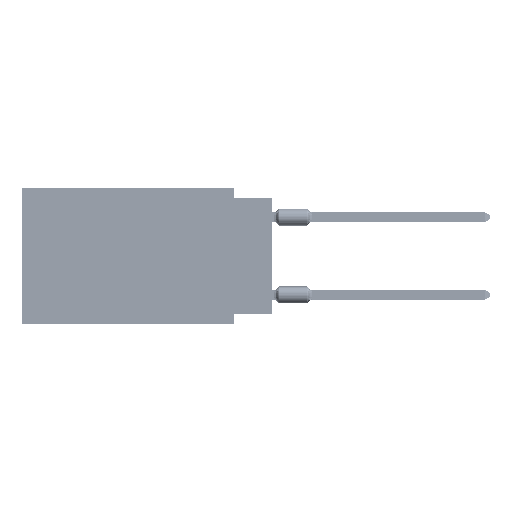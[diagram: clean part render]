
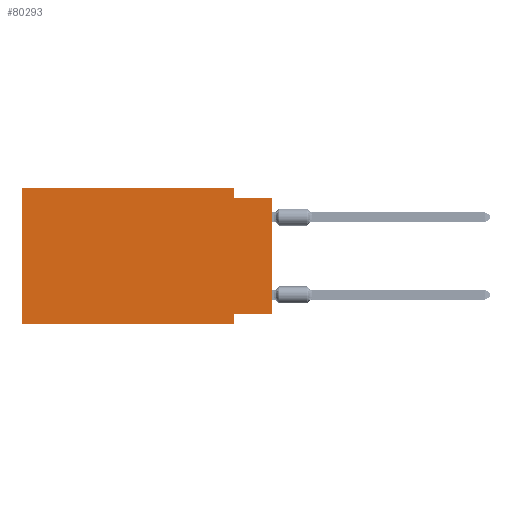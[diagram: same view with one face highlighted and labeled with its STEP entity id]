
A CAD part, left-side view. The second image highlights one B-rep face of the part: STEP entity #80293.
In plain terms, the highlighted planar face has unit normal (-1, 0, 0).
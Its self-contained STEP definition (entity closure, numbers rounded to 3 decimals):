
#221 = VECTOR ( 'NONE', #96902, 1000. ) ;
#2174 = VECTOR ( 'NONE', #97692, 1000. ) ;
#6761 = VERTEX_POINT ( 'NONE', #19589 ) ;
#8103 = VECTOR ( 'NONE', #70620, 1000. ) ;
#14086 = VERTEX_POINT ( 'NONE', #97853 ) ;
#14145 = EDGE_CURVE ( 'NONE', #23805, #6761, #61115, .T. ) ;
#17122 = CARTESIAN_POINT ( 'NONE',  ( 0., 16.383, -8.89 ) ) ;
#18074 = LINE ( 'NONE', #89787, #221 ) ;
#19589 = CARTESIAN_POINT ( 'NONE',  ( 0., 0., -0.635 ) ) ;
#19713 = LINE ( 'NONE', #30351, #54104 ) ;
#20325 = VERTEX_POINT ( 'NONE', #75668 ) ;
#23805 = VERTEX_POINT ( 'NONE', #88198 ) ;
#24097 = VECTOR ( 'NONE', #26695, 1000. ) ;
#25857 = ORIENTED_EDGE ( 'NONE', *, *, #102292, .F. ) ;
#26695 = DIRECTION ( 'NONE',  ( 0., -1., 0. ) ) ;
#28263 = DIRECTION ( 'NONE',  ( 0., 0., -1. ) ) ;
#29435 = LINE ( 'NONE', #92251, #42464 ) ;
#29451 = PLANE ( 'NONE',  #115308 ) ;
#30351 = CARTESIAN_POINT ( 'NONE',  ( 0., 0., -0.635 ) ) ;
#30402 = ORIENTED_EDGE ( 'NONE', *, *, #72761, .F. ) ;
#30609 = FACE_OUTER_BOUND ( 'NONE', #73069, .T. ) ;
#32565 = LINE ( 'NONE', #17122, #2174 ) ;
#32750 = ORIENTED_EDGE ( 'NONE', *, *, #60260, .T. ) ;
#37988 = DIRECTION ( 'NONE',  ( 0., 0., 1. ) ) ;
#38180 = VECTOR ( 'NONE', #37988, 1000. ) ;
#39143 = LINE ( 'NONE', #83614, #38180 ) ;
#40849 = EDGE_CURVE ( 'NONE', #14086, #113903, #72305, .T. ) ;
#42464 = VECTOR ( 'NONE', #28263, 1000. ) ;
#42532 = VECTOR ( 'NONE', #68549, 1000. ) ;
#46950 = DIRECTION ( 'NONE',  ( 0., -1., 0. ) ) ;
#48332 = CARTESIAN_POINT ( 'NONE',  ( 0., 16.383, -8.89 ) ) ;
#49326 = ORIENTED_EDGE ( 'NONE', *, *, #14145, .T. ) ;
#52803 = CARTESIAN_POINT ( 'NONE',  ( 0., 0., 0. ) ) ;
#54104 = VECTOR ( 'NONE', #46950, 1000. ) ;
#54745 = VERTEX_POINT ( 'NONE', #115375 ) ;
#60170 = DIRECTION ( 'NONE',  ( 0., 0., -1. ) ) ;
#60260 = EDGE_CURVE ( 'NONE', #61807, #54745, #32565, .T. ) ;
#60377 = VERTEX_POINT ( 'NONE', #100279 ) ;
#61115 = LINE ( 'NONE', #52803, #8103 ) ;
#61807 = VERTEX_POINT ( 'NONE', #48332 ) ;
#65578 = DIRECTION ( 'NONE',  ( 1., 0., 0. ) ) ;
#66745 = CARTESIAN_POINT ( 'NONE',  ( 0., 16.383, 0. ) ) ;
#68549 = DIRECTION ( 'NONE',  ( 0., 1., 0. ) ) ;
#70308 = LINE ( 'NONE', #106430, #42532 ) ;
#70620 = DIRECTION ( 'NONE',  ( 0., 0., 1. ) ) ;
#72305 = LINE ( 'NONE', #107853, #24097 ) ;
#72537 = ORIENTED_EDGE ( 'NONE', *, *, #96953, .F. ) ;
#72761 = EDGE_CURVE ( 'NONE', #23805, #60377, #70308, .T. ) ;
#73069 = EDGE_LOOP ( 'NONE', ( #49326, #25857, #72537, #75084, #108240, #32750, #100938, #30402 ) ) ;
#75084 = ORIENTED_EDGE ( 'NONE', *, *, #40849, .F. ) ;
#75668 = CARTESIAN_POINT ( 'NONE',  ( 0., 2.54, -0.635 ) ) ;
#80293 = ADVANCED_FACE ( 'NONE', ( #30609 ), #29451, .F. ) ;
#83614 = CARTESIAN_POINT ( 'NONE',  ( 0., 16.383, 0. ) ) ;
#84931 = EDGE_CURVE ( 'NONE', #61807, #14086, #39143, .T. ) ;
#88198 = CARTESIAN_POINT ( 'NONE',  ( 0., 0., -8.255 ) ) ;
#89787 = CARTESIAN_POINT ( 'NONE',  ( 0., 2.54, 0. ) ) ;
#92251 = CARTESIAN_POINT ( 'NONE',  ( 0., 2.54, -8.89 ) ) ;
#96902 = DIRECTION ( 'NONE',  ( 0., 0., -1. ) ) ;
#96953 = EDGE_CURVE ( 'NONE', #113903, #20325, #18074, .T. ) ;
#97692 = DIRECTION ( 'NONE',  ( 0., -1., 0. ) ) ;
#97853 = CARTESIAN_POINT ( 'NONE',  ( 0., 16.383, 0. ) ) ;
#98955 = EDGE_CURVE ( 'NONE', #60377, #54745, #29435, .T. ) ;
#100279 = CARTESIAN_POINT ( 'NONE',  ( 0., 2.54, -8.255 ) ) ;
#100938 = ORIENTED_EDGE ( 'NONE', *, *, #98955, .F. ) ;
#102292 = EDGE_CURVE ( 'NONE', #20325, #6761, #19713, .T. ) ;
#105617 = CARTESIAN_POINT ( 'NONE',  ( 0., 2.54, 0. ) ) ;
#106430 = CARTESIAN_POINT ( 'NONE',  ( 0., 0., -8.255 ) ) ;
#107853 = CARTESIAN_POINT ( 'NONE',  ( 0., 16.383, 0. ) ) ;
#108240 = ORIENTED_EDGE ( 'NONE', *, *, #84931, .F. ) ;
#113903 = VERTEX_POINT ( 'NONE', #105617 ) ;
#115308 = AXIS2_PLACEMENT_3D ( 'NONE', #66745, #65578, #60170 ) ;
#115375 = CARTESIAN_POINT ( 'NONE',  ( 0., 2.54, -8.89 ) ) ;
